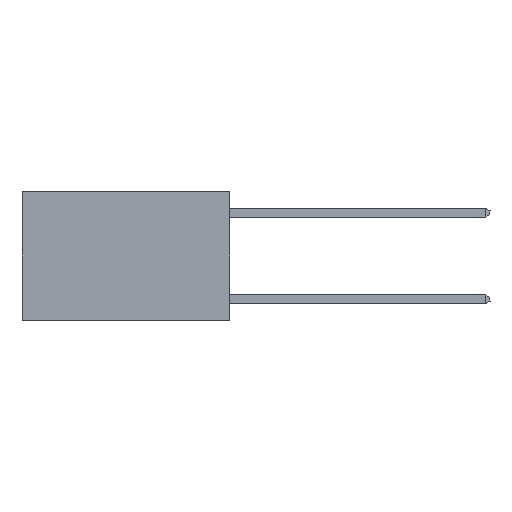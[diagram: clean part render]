
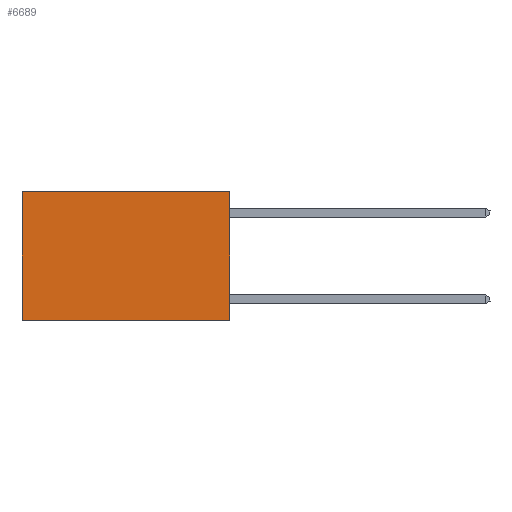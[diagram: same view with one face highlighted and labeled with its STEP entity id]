
A CAD part, left-side view. The second image highlights one B-rep face of the part: STEP entity #6689.
In plain terms, the highlighted planar face has unit normal (-1, 0, 0).
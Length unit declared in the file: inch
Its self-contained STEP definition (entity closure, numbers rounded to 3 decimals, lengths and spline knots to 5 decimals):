
#433 = DIRECTION ( 'NONE',  ( 0., 0., -1. ) ) ;
#648 = VERTEX_POINT ( 'NONE', #1169 ) ;
#657 = VECTOR ( 'NONE', #1622, 39.37008 ) ;
#667 = PLANE ( 'NONE',  #2818 ) ;
#1057 = LINE ( 'NONE', #4111, #5954 ) ;
#1169 = CARTESIAN_POINT ( 'NONE',  ( 0.2625, 0.6, 0. ) ) ;
#1489 = LINE ( 'NONE', #2991, #2482 ) ;
#1578 = EDGE_CURVE ( 'NONE', #3434, #9421, #1057, .T. ) ;
#1622 = DIRECTION ( 'NONE',  ( 0., 1., 0. ) ) ;
#1636 = VECTOR ( 'NONE', #1973, 39.37008 ) ;
#1647 = EDGE_CURVE ( 'NONE', #648, #2398, #7937, .T. ) ;
#1973 = DIRECTION ( 'NONE',  ( 0., 0., -1. ) ) ;
#2084 = ORIENTED_EDGE ( 'NONE', *, *, #1578, .F. ) ;
#2398 = VERTEX_POINT ( 'NONE', #7026 ) ;
#2482 = VECTOR ( 'NONE', #7450, 39.37008 ) ;
#2692 = CARTESIAN_POINT ( 'NONE',  ( 0.2625, 0., 0. ) ) ;
#2818 = AXIS2_PLACEMENT_3D ( 'NONE', #8791, #8880, #7384 ) ;
#2991 = CARTESIAN_POINT ( 'NONE',  ( 0.2625, 0., -0.37 ) ) ;
#3434 = VERTEX_POINT ( 'NONE', #2692 ) ;
#3664 = CARTESIAN_POINT ( 'NONE',  ( 0.2625, 0., 0. ) ) ;
#4111 = CARTESIAN_POINT ( 'NONE',  ( 0.2625, 0., 0. ) ) ;
#5038 = ORIENTED_EDGE ( 'NONE', *, *, #1647, .T. ) ;
#5271 = CARTESIAN_POINT ( 'NONE',  ( 0.2625, 0., -0.37 ) ) ;
#5954 = VECTOR ( 'NONE', #433, 39.37008 ) ;
#6662 = ORIENTED_EDGE ( 'NONE', *, *, #9055, .F. ) ;
#6689 = ADVANCED_FACE ( 'NONE', ( #8014 ), #667, .F. ) ;
#7026 = CARTESIAN_POINT ( 'NONE',  ( 0.2625, 0.6, -0.37 ) ) ;
#7346 = ORIENTED_EDGE ( 'NONE', *, *, #9437, .T. ) ;
#7384 = DIRECTION ( 'NONE',  ( 0., 0., -1. ) ) ;
#7450 = DIRECTION ( 'NONE',  ( 0., 1., 0. ) ) ;
#7937 = LINE ( 'NONE', #8714, #1636 ) ;
#8014 = FACE_OUTER_BOUND ( 'NONE', #9317, .T. ) ;
#8714 = CARTESIAN_POINT ( 'NONE',  ( 0.2625, 0.6, 0. ) ) ;
#8791 = CARTESIAN_POINT ( 'NONE',  ( 0.2625, 0., 0. ) ) ;
#8841 = LINE ( 'NONE', #3664, #657 ) ;
#8880 = DIRECTION ( 'NONE',  ( 1., 0., 0. ) ) ;
#9055 = EDGE_CURVE ( 'NONE', #9421, #2398, #1489, .T. ) ;
#9317 = EDGE_LOOP ( 'NONE', ( #5038, #6662, #2084, #7346 ) ) ;
#9421 = VERTEX_POINT ( 'NONE', #5271 ) ;
#9437 = EDGE_CURVE ( 'NONE', #3434, #648, #8841, .T. ) ;
